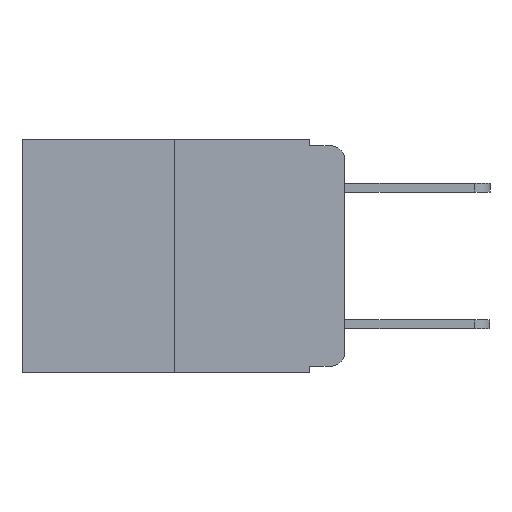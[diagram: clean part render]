
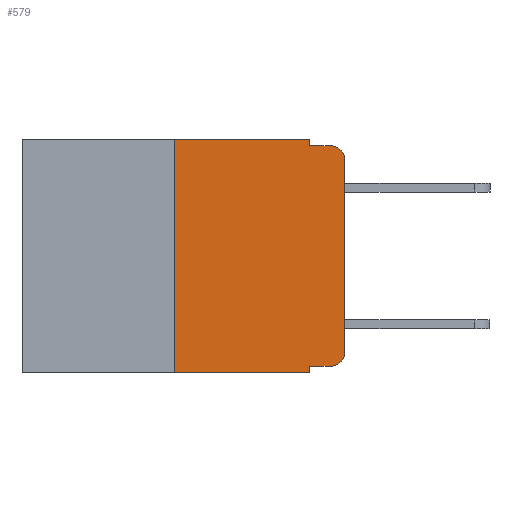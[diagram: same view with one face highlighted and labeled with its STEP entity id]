
A CAD part, left-side view. The second image highlights one B-rep face of the part: STEP entity #579.
In plain terms, the highlighted planar face has unit normal (-1, 0, 0).
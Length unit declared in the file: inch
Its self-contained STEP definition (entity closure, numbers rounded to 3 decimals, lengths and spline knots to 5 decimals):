
#130 = LINE ( 'NONE', #8935, #345 ) ;
#313 = DIRECTION ( 'NONE',  ( 0., 0., 1. ) ) ;
#345 = VECTOR ( 'NONE', #313, 39.37008 ) ;
#508 = EDGE_CURVE ( 'NONE', #5052, #9153, #8644, .T. ) ;
#554 = EDGE_CURVE ( 'NONE', #6222, #6470, #7692, .T. ) ;
#579 = ADVANCED_FACE ( 'NONE', ( #3009 ), #2053, .F. ) ;
#754 = CARTESIAN_POINT ( 'NONE',  ( 0., 0., 0. ) ) ;
#937 = DIRECTION ( 'NONE',  ( 0., 0., 1. ) ) ;
#1009 = LINE ( 'NONE', #11558, #3788 ) ;
#1490 = VERTEX_POINT ( 'NONE', #5959 ) ;
#1659 = EDGE_CURVE ( 'NONE', #5052, #6393, #5639, .T. ) ;
#2053 = PLANE ( 'NONE',  #8849 ) ;
#2064 = DIRECTION ( 'NONE',  ( 0., 0., -1. ) ) ;
#2154 = CARTESIAN_POINT ( 'NONE',  ( 0., 0.25, 0. ) ) ;
#2295 = CARTESIAN_POINT ( 'NONE',  ( 0., 0.02, -0.333 ) ) ;
#2614 = VERTEX_POINT ( 'NONE', #2154 ) ;
#2882 = LINE ( 'NONE', #5862, #7582 ) ;
#2883 = CARTESIAN_POINT ( 'NONE',  ( 0., 0.051, -0.01 ) ) ;
#3002 = CARTESIAN_POINT ( 'NONE',  ( 0., 0.02, -0.01 ) ) ;
#3009 = FACE_OUTER_BOUND ( 'NONE', #11428, .T. ) ;
#3076 = DIRECTION ( 'NONE',  ( 1., 0., 0. ) ) ;
#3086 = DIRECTION ( 'NONE',  ( -1., 0., 0. ) ) ;
#3250 = ORIENTED_EDGE ( 'NONE', *, *, #554, .F. ) ;
#3266 = ORIENTED_EDGE ( 'NONE', *, *, #7322, .T. ) ;
#3459 = CARTESIAN_POINT ( 'NONE',  ( 0., 0.02, -0.03 ) ) ;
#3608 = VECTOR ( 'NONE', #6756, 39.37008 ) ;
#3732 = CARTESIAN_POINT ( 'NONE',  ( 0., 0., -0.03 ) ) ;
#3788 = VECTOR ( 'NONE', #9738, 39.37008 ) ;
#3805 = EDGE_CURVE ( 'NONE', #4684, #6470, #11188, .T. ) ;
#3822 = ORIENTED_EDGE ( 'NONE', *, *, #1659, .F. ) ;
#3902 = CARTESIAN_POINT ( 'NONE',  ( 0., 0.051, -0.01 ) ) ;
#3907 = DIRECTION ( 'NONE',  ( 0., -1., 0. ) ) ;
#4348 = EDGE_CURVE ( 'NONE', #1490, #4684, #9620, .T. ) ;
#4460 = EDGE_CURVE ( 'NONE', #7140, #2614, #130, .T. ) ;
#4538 = DIRECTION ( 'NONE',  ( -1., 0., 0. ) ) ;
#4684 = VERTEX_POINT ( 'NONE', #3732 ) ;
#4895 = ORIENTED_EDGE ( 'NONE', *, *, #6872, .T. ) ;
#5052 = VERTEX_POINT ( 'NONE', #5775 ) ;
#5256 = CIRCLE ( 'NONE', #8702, 0.02 ) ;
#5418 = VERTEX_POINT ( 'NONE', #8480 ) ;
#5501 = CARTESIAN_POINT ( 'NONE',  ( 0., 0.25, -0.343 ) ) ;
#5639 = LINE ( 'NONE', #8347, #6101 ) ;
#5775 = CARTESIAN_POINT ( 'NONE',  ( 0., 0.051, -0.333 ) ) ;
#5787 = AXIS2_PLACEMENT_3D ( 'NONE', #3459, #4538, #12011 ) ;
#5862 = CARTESIAN_POINT ( 'NONE',  ( 0., 0.051, 0. ) ) ;
#5959 = CARTESIAN_POINT ( 'NONE',  ( 0., 0., -0.313 ) ) ;
#6101 = VECTOR ( 'NONE', #8413, 39.37008 ) ;
#6222 = VERTEX_POINT ( 'NONE', #3902 ) ;
#6393 = VERTEX_POINT ( 'NONE', #8513 ) ;
#6470 = VERTEX_POINT ( 'NONE', #3002 ) ;
#6670 = EDGE_CURVE ( 'NONE', #2614, #5418, #10229, .T. ) ;
#6689 = DIRECTION ( 'NONE',  ( 0., 0., -1. ) ) ;
#6756 = DIRECTION ( 'NONE',  ( 0., -1., 0. ) ) ;
#6779 = ORIENTED_EDGE ( 'NONE', *, *, #4460, .F. ) ;
#6872 = EDGE_CURVE ( 'NONE', #7140, #6393, #1009, .T. ) ;
#6943 = CARTESIAN_POINT ( 'NONE',  ( 0., 0.473, 0. ) ) ;
#7140 = VERTEX_POINT ( 'NONE', #5501 ) ;
#7322 = EDGE_CURVE ( 'NONE', #9153, #1490, #5256, .T. ) ;
#7582 = VECTOR ( 'NONE', #6689, 39.37008 ) ;
#7665 = ORIENTED_EDGE ( 'NONE', *, *, #508, .T. ) ;
#7692 = LINE ( 'NONE', #2883, #3608 ) ;
#8347 = CARTESIAN_POINT ( 'NONE',  ( 0., 0.051, 0. ) ) ;
#8413 = DIRECTION ( 'NONE',  ( 0., 0., -1. ) ) ;
#8480 = CARTESIAN_POINT ( 'NONE',  ( 0., 0.051, 0. ) ) ;
#8513 = CARTESIAN_POINT ( 'NONE',  ( 0., 0.051, -0.343 ) ) ;
#8644 = LINE ( 'NONE', #9459, #11229 ) ;
#8702 = AXIS2_PLACEMENT_3D ( 'NONE', #10882, #3086, #2064 ) ;
#8849 = AXIS2_PLACEMENT_3D ( 'NONE', #6943, #3076, #8897 ) ;
#8897 = DIRECTION ( 'NONE',  ( 0., 0., -1. ) ) ;
#8935 = CARTESIAN_POINT ( 'NONE',  ( 0., 0.25, 0. ) ) ;
#9153 = VERTEX_POINT ( 'NONE', #2295 ) ;
#9166 = ORIENTED_EDGE ( 'NONE', *, *, #3805, .T. ) ;
#9459 = CARTESIAN_POINT ( 'NONE',  ( 0., 0.051, -0.333 ) ) ;
#9620 = LINE ( 'NONE', #754, #10819 ) ;
#9738 = DIRECTION ( 'NONE',  ( 0., -1., 0. ) ) ;
#10124 = ORIENTED_EDGE ( 'NONE', *, *, #4348, .T. ) ;
#10229 = LINE ( 'NONE', #11996, #10862 ) ;
#10326 = EDGE_CURVE ( 'NONE', #5418, #6222, #2882, .T. ) ;
#10344 = ORIENTED_EDGE ( 'NONE', *, *, #10326, .F. ) ;
#10819 = VECTOR ( 'NONE', #937, 39.37008 ) ;
#10862 = VECTOR ( 'NONE', #12064, 39.37008 ) ;
#10882 = CARTESIAN_POINT ( 'NONE',  ( 0., 0.02, -0.313 ) ) ;
#10970 = ORIENTED_EDGE ( 'NONE', *, *, #6670, .F. ) ;
#11188 = CIRCLE ( 'NONE', #5787, 0.02 ) ;
#11229 = VECTOR ( 'NONE', #3907, 39.37008 ) ;
#11428 = EDGE_LOOP ( 'NONE', ( #10124, #9166, #3250, #10344, #10970, #6779, #4895, #3822, #7665, #3266 ) ) ;
#11558 = CARTESIAN_POINT ( 'NONE',  ( 0., 0.473, -0.343 ) ) ;
#11996 = CARTESIAN_POINT ( 'NONE',  ( 0., 0.473, 0. ) ) ;
#12011 = DIRECTION ( 'NONE',  ( 0., 0., -1. ) ) ;
#12064 = DIRECTION ( 'NONE',  ( 0., -1., 0. ) ) ;
